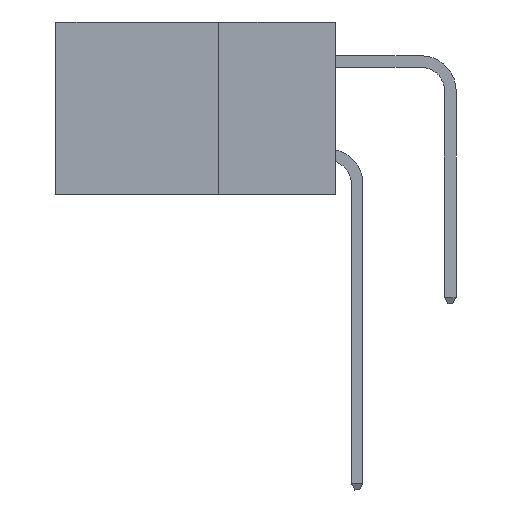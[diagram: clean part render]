
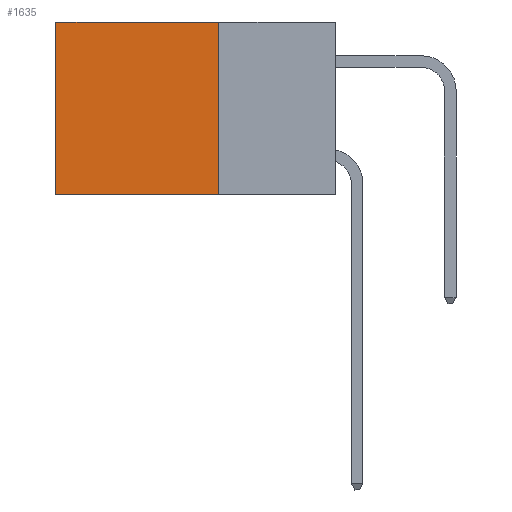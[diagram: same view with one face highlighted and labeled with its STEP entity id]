
A CAD part, left-side view. The second image highlights one B-rep face of the part: STEP entity #1635.
In plain terms, the highlighted planar face has unit normal (-1, 0, 0).
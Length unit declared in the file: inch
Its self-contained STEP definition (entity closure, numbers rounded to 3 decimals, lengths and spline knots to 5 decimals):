
#566 = FACE_OUTER_BOUND ( 'NONE', #10018, .T. ) ;
#792 = ORIENTED_EDGE ( 'NONE', *, *, #2978, .F. ) ;
#1289 = LINE ( 'NONE', #20413, #28678 ) ;
#1635 = ADVANCED_FACE ( 'NONE', ( #566 ), #32032, .F. ) ;
#2272 = CARTESIAN_POINT ( 'NONE',  ( 0.2875, 0.25, 0. ) ) ;
#2364 = DIRECTION ( 'NONE',  ( 0., 0., -1. ) ) ;
#2388 = LINE ( 'NONE', #17247, #35624 ) ;
#2550 = VERTEX_POINT ( 'NONE', #11205 ) ;
#2978 = EDGE_CURVE ( 'NONE', #28756, #24956, #7406, .T. ) ;
#3258 = ORIENTED_EDGE ( 'NONE', *, *, #34674, .T. ) ;
#4417 = ORIENTED_EDGE ( 'NONE', *, *, #21197, .F. ) ;
#5236 = CARTESIAN_POINT ( 'NONE',  ( 0.2875, 0.6, 0. ) ) ;
#6468 = CARTESIAN_POINT ( 'NONE',  ( 0.2875, 0.25, 0. ) ) ;
#7406 = LINE ( 'NONE', #27985, #29975 ) ;
#8973 = EDGE_CURVE ( 'NONE', #28756, #2550, #2388, .T. ) ;
#10018 = EDGE_LOOP ( 'NONE', ( #3258, #4417, #792, #35850 ) ) ;
#10582 = LINE ( 'NONE', #5236, #20913 ) ;
#11205 = CARTESIAN_POINT ( 'NONE',  ( 0.2875, 0.6, 0. ) ) ;
#12559 = AXIS2_PLACEMENT_3D ( 'NONE', #6468, #29554, #32578 ) ;
#16732 = DIRECTION ( 'NONE',  ( 0., 0., -1. ) ) ;
#17067 = CARTESIAN_POINT ( 'NONE',  ( 0.2875, 0.25, -0.37 ) ) ;
#17247 = CARTESIAN_POINT ( 'NONE',  ( 0.2875, 0.25, 0. ) ) ;
#18317 = CARTESIAN_POINT ( 'NONE',  ( 0.2875, 0.6, -0.37 ) ) ;
#20413 = CARTESIAN_POINT ( 'NONE',  ( 0.2875, 0.25, -0.37 ) ) ;
#20913 = VECTOR ( 'NONE', #2364, 39.37008 ) ;
#21197 = EDGE_CURVE ( 'NONE', #24956, #25535, #1289, .T. ) ;
#24956 = VERTEX_POINT ( 'NONE', #17067 ) ;
#25535 = VERTEX_POINT ( 'NONE', #18317 ) ;
#27985 = CARTESIAN_POINT ( 'NONE',  ( 0.2875, 0.25, 0. ) ) ;
#28678 = VECTOR ( 'NONE', #30085, 39.37008 ) ;
#28756 = VERTEX_POINT ( 'NONE', #2272 ) ;
#29064 = DIRECTION ( 'NONE',  ( 0., 1., 0. ) ) ;
#29554 = DIRECTION ( 'NONE',  ( 1., 0., 0. ) ) ;
#29975 = VECTOR ( 'NONE', #16732, 39.37008 ) ;
#30085 = DIRECTION ( 'NONE',  ( 0., 1., 0. ) ) ;
#32032 = PLANE ( 'NONE',  #12559 ) ;
#32578 = DIRECTION ( 'NONE',  ( 0., 0., -1. ) ) ;
#34674 = EDGE_CURVE ( 'NONE', #2550, #25535, #10582, .T. ) ;
#35624 = VECTOR ( 'NONE', #29064, 39.37008 ) ;
#35850 = ORIENTED_EDGE ( 'NONE', *, *, #8973, .T. ) ;
